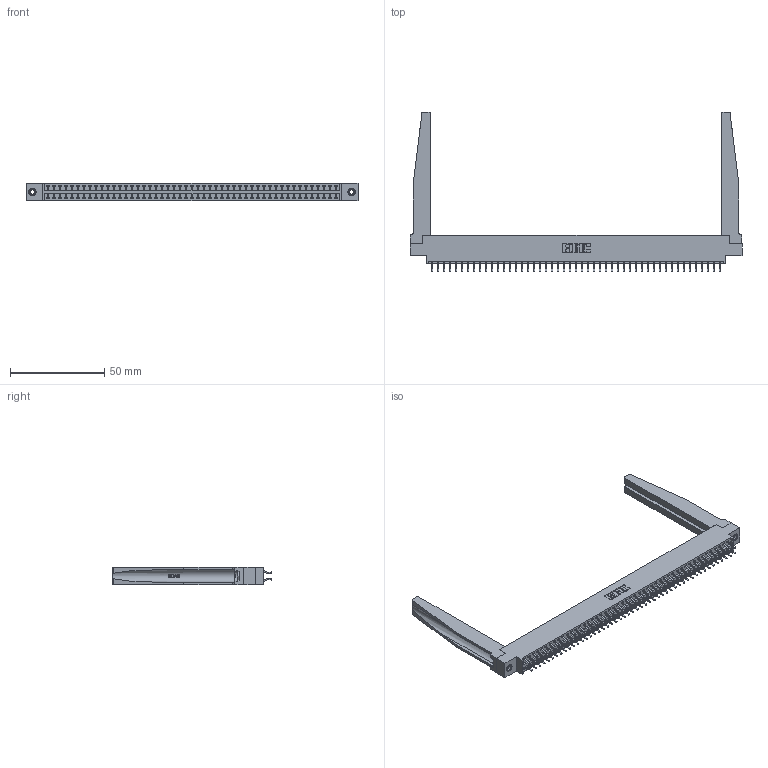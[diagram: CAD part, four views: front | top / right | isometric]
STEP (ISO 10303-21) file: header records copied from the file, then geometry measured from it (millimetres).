
FILE_DESCRIPTION (( 'STEP AP203' ), '1' );
FILE_NAME ('396-098-556-878.STEP', '2019-11-02T17:16:09', ( '' ), ( '' ), 'SwSTEP 2.0', 'SolidWorks 2016', '' );
FILE_SCHEMA (( 'CONFIG_CONTROL_DESIGN' ));
Length unit declared in the file: inch
Products named in the file (5): 396-098-556-878; 346 Part_0.170 Offset - 0.156 Dia-TH; 345-292-001_556 Tail; 346-220-078_345-220-078; 345-250-001_345-250-001-102
Assembly tree (103 placements, depth 2):
  396-098-556-878
    346 Part_0.170 Offset - 0.156 Dia-TH
    345-292-001_556 Tail  x98
    346-220-078_345-220-078  x2
    345-250-001_345-250-001-102  x2
Bounding box: 176.15 x 84.84 x 9.4 mm (x, y, z)
Volume: 23981.4 mm3; surface area: 30203.5 mm2
Topology: 103 solids, 103 shells, 6044 faces, 17903 edges, 11794 vertices
Faces by surface type: plane 4044, cylinder 1948, bspline 36, cone 12, torus 4
Entity records: 36136 total; most frequent: CARTESIAN_POINT 6899, ORIENTED_EDGE 5710, DIRECTION 5105, EDGE_CURVE 2855, VECTOR 2425, LINE 2425, VERTEX_POINT 1896, AXIS2_PLACEMENT_3D 1340
